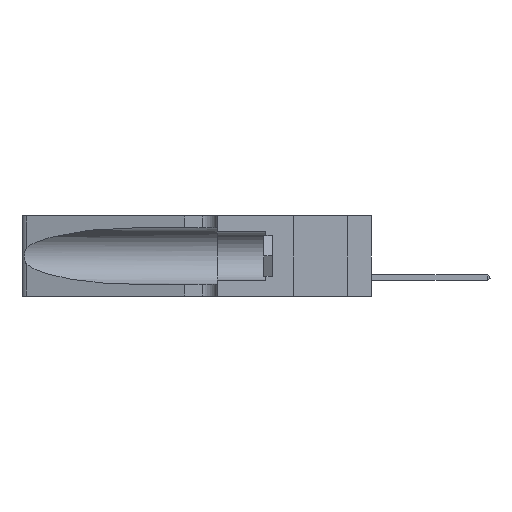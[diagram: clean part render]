
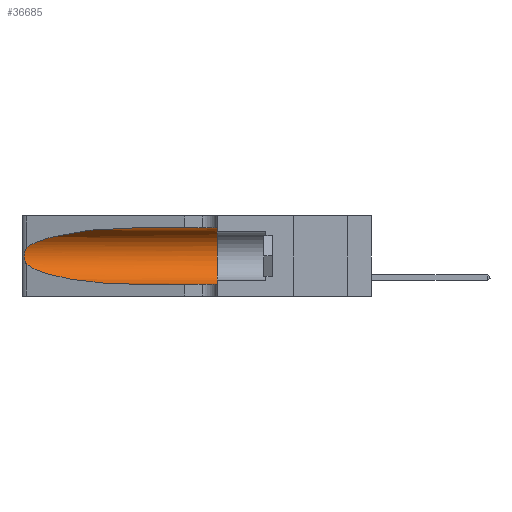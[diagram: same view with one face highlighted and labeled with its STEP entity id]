
A CAD part, left-side view. The second image highlights one B-rep face of the part: STEP entity #36685.
In plain terms, the highlighted cylindrical face has radius 3.308 mm (diameter 6.617 mm), a partial arc.
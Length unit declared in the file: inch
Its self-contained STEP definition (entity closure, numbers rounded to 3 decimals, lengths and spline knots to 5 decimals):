
#1289 = EDGE_CURVE ( 'NONE', #36591, #11351, #16105, .T. ) ;
#2339 = CARTESIAN_POINT ( 'NONE',  ( 0.25487, 1.22718, 0.22369 ) ) ;
#2458 = DIRECTION ( 'NONE',  ( 0., 0., 1. ) ) ;
#3436 = EDGE_LOOP ( 'NONE', ( #26627, #4864, #6807, #28041, #30883, #20538 ) ) ;
#3590 = VECTOR ( 'NONE', #12623, 39.37008 ) ;
#4191 = CARTESIAN_POINT ( 'NONE',  ( 0.1305, 0.72297, 0.05475 ) ) ;
#4638 = LINE ( 'NONE', #5850, #3590 ) ;
#4864 = ORIENTED_EDGE ( 'NONE', *, *, #5255, .T. ) ;
#5023 = AXIS2_PLACEMENT_3D ( 'NONE', #8764, #17802, #2458 ) ;
#5062 = CARTESIAN_POINT ( 'NONE',  ( 0.25856, 1.23593, 0.16098 ) ) ;
#5255 = EDGE_CURVE ( 'NONE', #11351, #27576, #40863, .T. ) ;
#5329 = CARTESIAN_POINT ( 'NONE',  ( 0.25487, 1.22718, 0.14631 ) ) ;
#5850 = CARTESIAN_POINT ( 'NONE',  ( 0.1305, 1.61858, 0.05475 ) ) ;
#6807 = ORIENTED_EDGE ( 'NONE', *, *, #16831, .T. ) ;
#7528 = CYLINDRICAL_SURFACE ( 'NONE', #13480, 0.13025 ) ;
#7997 = CARTESIAN_POINT ( 'NONE',  ( 0.25487, 1.22718, 0.22369 ) ) ;
#8412 = CARTESIAN_POINT ( 'NONE',  ( 0.25487, 1.22718, 0.22369 ) ) ;
#8495 = VERTEX_POINT ( 'NONE', #29312 ) ;
#8684 = CARTESIAN_POINT ( 'NONE',  ( 0.25787, 1.23484, 0.2124 ) ) ;
#8764 = CARTESIAN_POINT ( 'NONE',  ( 0.1305, 0.35, 0.185 ) ) ;
#8952 = CARTESIAN_POINT ( 'NONE',  ( 0.1305, 0.35, 0.31525 ) ) ;
#10755 = CARTESIAN_POINT ( 'NONE',  ( 0.18966, 0.96281, 0.05475 ) ) ;
#11178 = DIRECTION ( 'NONE',  ( 0., -1., 0. ) ) ;
#11351 = VERTEX_POINT ( 'NONE', #7997 ) ;
#11461 = CARTESIAN_POINT ( 'NONE',  ( 0.25555, 1.22993, 0.14849 ) ) ;
#11482 = DIRECTION ( 'NONE',  ( 0., -1., 0. ) ) ;
#11594 = CARTESIAN_POINT ( 'NONE',  ( 0.25555, 1.22994, 0.2215 ) ) ;
#11724 = CARTESIAN_POINT ( 'NONE',  ( 0.25639, 1.23184, 0.21858 ) ) ;
#11861 = CARTESIAN_POINT ( 'NONE',  ( 0.26017, 1.23833, 0.17102 ) ) ;
#12046 = EDGE_CURVE ( 'NONE', #36591, #22111, #41079, .T. ) ;
#12623 = DIRECTION ( 'NONE',  ( 0., -1., 0. ) ) ;
#13480 = AXIS2_PLACEMENT_3D ( 'NONE', #20844, #11482, #17889 ) ;
#15411 =( BOUNDED_CURVE ( )  B_SPLINE_CURVE ( 3, ( #33420, #16861, #10755, #4191 ),
 .UNSPECIFIED., .F., .T. ) 
 B_SPLINE_CURVE_WITH_KNOTS ( ( 4, 4 ),
 ( 3.44316, 4.71239 ),
 .UNSPECIFIED. ) 
 CURVE ( )  GEOMETRIC_REPRESENTATION_ITEM ( )  RATIONAL_B_SPLINE_CURVE ( ( 1., 0.87, 0.87, 1. ) ) 
 REPRESENTATION_ITEM ( '' )  );
#16105 =( BOUNDED_CURVE ( )  B_SPLINE_CURVE ( 3, ( #21187, #27631, #30086, #2339 ),
 .UNSPECIFIED., .F., .T. ) 
 B_SPLINE_CURVE_WITH_KNOTS ( ( 4, 4 ),
 ( 1.5708, 2.84003 ),
 .UNSPECIFIED. ) 
 CURVE ( )  GEOMETRIC_REPRESENTATION_ITEM ( )  RATIONAL_B_SPLINE_CURVE ( ( 1., 0.87, 0.87, 1. ) ) 
 REPRESENTATION_ITEM ( '' )  );
#16831 = EDGE_CURVE ( 'NONE', #27576, #8495, #15411, .T. ) ;
#16861 = CARTESIAN_POINT ( 'NONE',  ( 0.2373, 1.15595, 0.08982 ) ) ;
#17140 = EDGE_CURVE ( 'NONE', #22111, #34839, #36100, .T. ) ;
#17565 = CARTESIAN_POINT ( 'NONE',  ( 0.1305, 1.61858, 0.31525 ) ) ;
#17802 = DIRECTION ( 'NONE',  ( 0., 1., 0. ) ) ;
#17889 = DIRECTION ( 'NONE',  ( 0., 0., -1. ) ) ;
#20538 = ORIENTED_EDGE ( 'NONE', *, *, #12046, .F. ) ;
#20844 = CARTESIAN_POINT ( 'NONE',  ( 0.1305, 1.61858, 0.185 ) ) ;
#21108 = CARTESIAN_POINT ( 'NONE',  ( 0.26075, 1.23896, 0.178 ) ) ;
#21187 = CARTESIAN_POINT ( 'NONE',  ( 0.1305, 0.72297, 0.31525 ) ) ;
#22111 = VERTEX_POINT ( 'NONE', #8952 ) ;
#23626 = CARTESIAN_POINT ( 'NONE',  ( 0.1305, 0.35, 0.05475 ) ) ;
#25106 = FACE_OUTER_BOUND ( 'NONE', #3436, .T. ) ;
#26627 = ORIENTED_EDGE ( 'NONE', *, *, #1289, .T. ) ;
#27576 = VERTEX_POINT ( 'NONE', #38518 ) ;
#27631 = CARTESIAN_POINT ( 'NONE',  ( 0.18966, 0.96281, 0.31525 ) ) ;
#28041 = ORIENTED_EDGE ( 'NONE', *, *, #37622, .T. ) ;
#29312 = CARTESIAN_POINT ( 'NONE',  ( 0.1305, 0.72297, 0.05475 ) ) ;
#30086 = CARTESIAN_POINT ( 'NONE',  ( 0.2373, 1.15595, 0.28018 ) ) ;
#30883 = ORIENTED_EDGE ( 'NONE', *, *, #17140, .F. ) ;
#32067 = VECTOR ( 'NONE', #11178, 39.37008 ) ;
#33420 = CARTESIAN_POINT ( 'NONE',  ( 0.25487, 1.22718, 0.14631 ) ) ;
#34238 = CARTESIAN_POINT ( 'NONE',  ( 0.25789, 1.23486, 0.15765 ) ) ;
#34375 = CARTESIAN_POINT ( 'NONE',  ( 0.26018, 1.23835, 0.19895 ) ) ;
#34839 = VERTEX_POINT ( 'NONE', #23626 ) ;
#36100 = CIRCLE ( 'NONE', #5023, 0.13025 ) ;
#36591 = VERTEX_POINT ( 'NONE', #39864 ) ;
#36685 = ADVANCED_FACE ( 'NONE', ( #25106 ), #7528, .F. ) ;
#37025 = CARTESIAN_POINT ( 'NONE',  ( 0.26075, 1.23896, 0.19203 ) ) ;
#37169 = CARTESIAN_POINT ( 'NONE',  ( 0.25639, 1.23186, 0.15144 ) ) ;
#37622 = EDGE_CURVE ( 'NONE', #8495, #34839, #4638, .T. ) ;
#38518 = CARTESIAN_POINT ( 'NONE',  ( 0.25487, 1.22718, 0.14631 ) ) ;
#39864 = CARTESIAN_POINT ( 'NONE',  ( 0.1305, 0.72297, 0.31525 ) ) ;
#40407 = CARTESIAN_POINT ( 'NONE',  ( 0.25854, 1.2359, 0.20912 ) ) ;
#40863 = B_SPLINE_CURVE_WITH_KNOTS ( 'NONE', 3,
 ( #8412, #11594, #11724, #8684, #40407, #34375, #37025, #21108, #11861, #5062, #34238, #37169, #11461, #5329 ),
 .UNSPECIFIED., .F., .F.,
 ( 4, 2, 2, 2, 2, 2, 4 ),
 ( 0., 0.00027, 0.00053, 0.00107, 0.0016, 0.00187, 0.00214 ),
 .UNSPECIFIED. ) ;
#41079 = LINE ( 'NONE', #17565, #32067 ) ;
